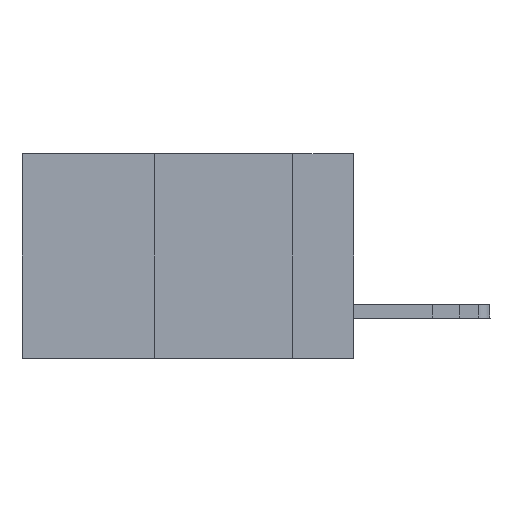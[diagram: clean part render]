
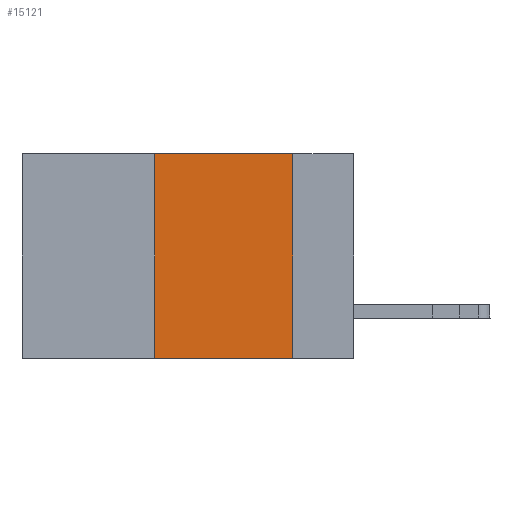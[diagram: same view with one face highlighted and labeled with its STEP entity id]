
A CAD part, left-side view. The second image highlights one B-rep face of the part: STEP entity #15121.
In plain terms, the highlighted planar face has unit normal (-1, 0, 0).
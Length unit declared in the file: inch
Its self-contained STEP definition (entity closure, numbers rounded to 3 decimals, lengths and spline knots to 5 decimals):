
#2423 = CARTESIAN_POINT ( 'NONE',  ( 0., 0.36, 0. ) ) ;
#3168 = VECTOR ( 'NONE', #3520, 39.37008 ) ;
#3355 = DIRECTION ( 'NONE',  ( 0., 0., -1. ) ) ;
#3485 = CARTESIAN_POINT ( 'NONE',  ( 0., 0.11, -0.37 ) ) ;
#3520 = DIRECTION ( 'NONE',  ( 0., -1., 0. ) ) ;
#3578 = CARTESIAN_POINT ( 'NONE',  ( 0., 0.36, 0. ) ) ;
#3753 = VECTOR ( 'NONE', #3355, 39.37008 ) ;
#4163 = VERTEX_POINT ( 'NONE', #14979 ) ;
#4414 = ORIENTED_EDGE ( 'NONE', *, *, #10755, .F. ) ;
#4860 = CARTESIAN_POINT ( 'NONE',  ( 0., 0.6, 0. ) ) ;
#4980 = DIRECTION ( 'NONE',  ( 1., 0., 0. ) ) ;
#5518 = LINE ( 'NONE', #24390, #3168 ) ;
#5942 = EDGE_CURVE ( 'NONE', #4163, #15276, #5518, .T. ) ;
#6109 = CARTESIAN_POINT ( 'NONE',  ( 0., 0.6, 0. ) ) ;
#8670 = VECTOR ( 'NONE', #13403, 39.37008 ) ;
#10131 = VERTEX_POINT ( 'NONE', #2423 ) ;
#10187 = EDGE_LOOP ( 'NONE', ( #4414, #20654, #24666, #21590 ) ) ;
#10755 = EDGE_CURVE ( 'NONE', #11502, #15276, #16682, .T. ) ;
#10854 = DIRECTION ( 'NONE',  ( 0., 0., 1. ) ) ;
#11502 = VERTEX_POINT ( 'NONE', #23803 ) ;
#13403 = DIRECTION ( 'NONE',  ( 0., -1., 0. ) ) ;
#14364 = VECTOR ( 'NONE', #10854, 39.37008 ) ;
#14559 = PLANE ( 'NONE',  #21201 ) ;
#14979 = CARTESIAN_POINT ( 'NONE',  ( 0., 0.36, -0.37 ) ) ;
#15121 = ADVANCED_FACE ( 'NONE', ( #22218 ), #14559, .F. ) ;
#15276 = VERTEX_POINT ( 'NONE', #3485 ) ;
#16682 = LINE ( 'NONE', #24351, #3753 ) ;
#16787 = LINE ( 'NONE', #3578, #14364 ) ;
#18029 = EDGE_CURVE ( 'NONE', #10131, #11502, #19331, .T. ) ;
#19331 = LINE ( 'NONE', #6109, #8670 ) ;
#19562 = EDGE_CURVE ( 'NONE', #4163, #10131, #16787, .T. ) ;
#20351 = DIRECTION ( 'NONE',  ( 0., 0., -1. ) ) ;
#20654 = ORIENTED_EDGE ( 'NONE', *, *, #18029, .F. ) ;
#21201 = AXIS2_PLACEMENT_3D ( 'NONE', #4860, #4980, #20351 ) ;
#21590 = ORIENTED_EDGE ( 'NONE', *, *, #5942, .T. ) ;
#22218 = FACE_OUTER_BOUND ( 'NONE', #10187, .T. ) ;
#23803 = CARTESIAN_POINT ( 'NONE',  ( 0., 0.11, 0. ) ) ;
#24351 = CARTESIAN_POINT ( 'NONE',  ( 0., 0.11, 0. ) ) ;
#24390 = CARTESIAN_POINT ( 'NONE',  ( 0., 0.6, -0.37 ) ) ;
#24666 = ORIENTED_EDGE ( 'NONE', *, *, #19562, .F. ) ;
